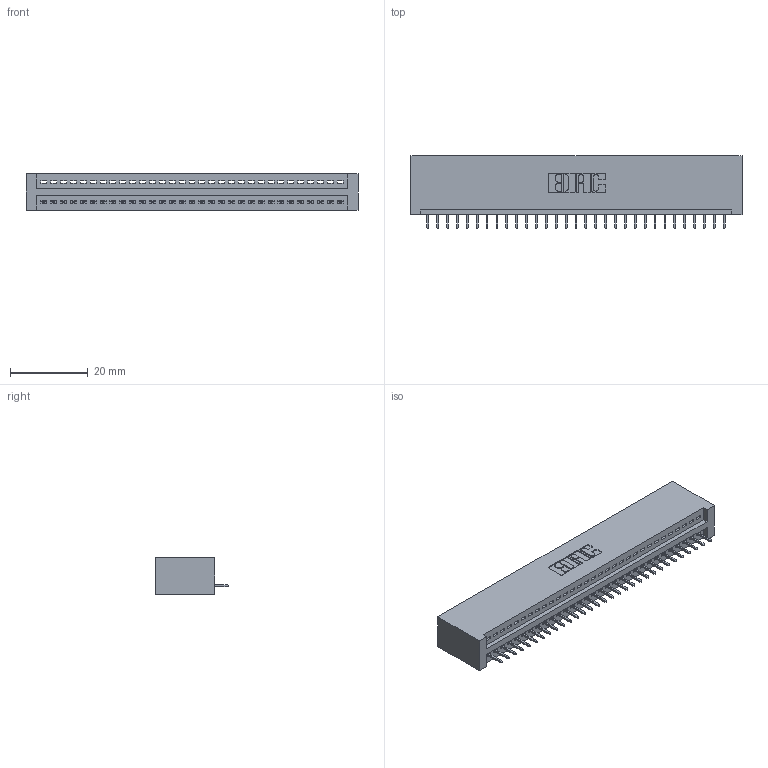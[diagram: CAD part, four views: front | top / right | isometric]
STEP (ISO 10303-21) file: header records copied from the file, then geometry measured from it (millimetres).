
FILE_DESCRIPTION (( 'STEP AP203' ), '1' );
FILE_NAME ('845-031-525-101.STEP', '2020-09-23T00:34:10', ( '' ), ( '' ), 'SwSTEP 2.0', 'SolidWorks 2020', '' );
FILE_SCHEMA (( 'CONFIG_CONTROL_DESIGN' ));
Length unit declared in the file: inch
Products named in the file (3): 845-031-525-101; 845 Part_No Mounting Lugs; 345-292-001_345-293-125
Assembly tree (32 placements, depth 2):
  845-031-525-101
    845 Part_No Mounting Lugs
    345-292-001_345-293-125  x31
Bounding box: 85.34 x 18.72 x 9.4 mm (x, y, z)
Volume: 8473.7 mm3; surface area: 10879.4 mm2
Topology: 32 solids, 32 shells, 2040 faces, 5897 edges, 3806 vertices
Faces by surface type: plane 1502, cylinder 538
Entity records: 24609 total; most frequent: CARTESIAN_POINT 4269, ORIENTED_EDGE 4234, DIRECTION 3739, EDGE_CURVE 2117, VECTOR 1873, LINE 1873, VERTEX_POINT 1406, AXIS2_PLACEMENT_3D 933
